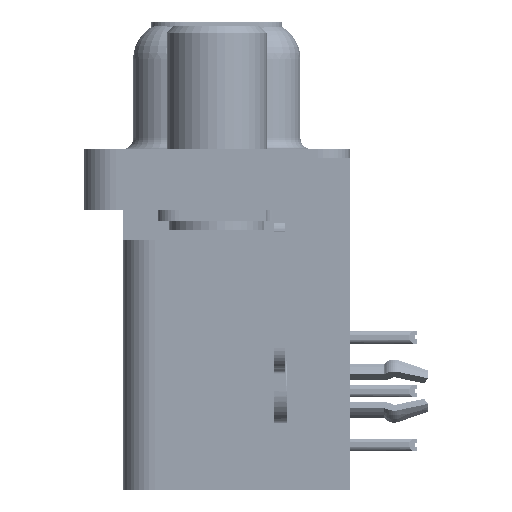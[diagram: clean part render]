
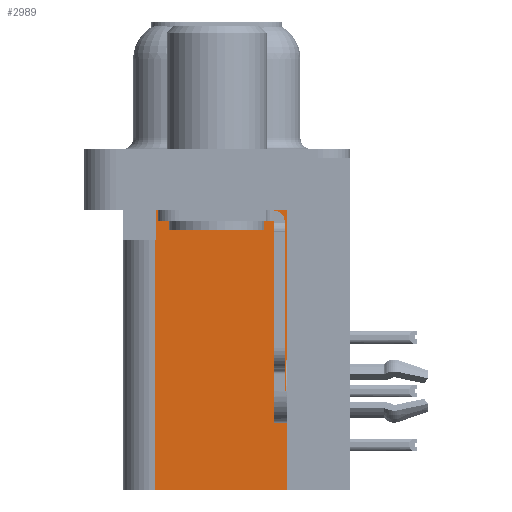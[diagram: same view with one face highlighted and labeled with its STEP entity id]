
A CAD part, left-side view. The second image highlights one B-rep face of the part: STEP entity #2989.
In plain terms, the highlighted planar face has unit normal (-1, 0, 0).
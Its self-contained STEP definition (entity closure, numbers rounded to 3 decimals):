
#494 = VECTOR ( 'NONE', #29950, 1000. ) ;
#585 = LINE ( 'NONE', #4386, #494 ) ;
#861 = CARTESIAN_POINT ( 'NONE',  ( 3.7, 2.895, -3.9 ) ) ;
#946 = CARTESIAN_POINT ( 'NONE',  ( 3.7, -3.295, -15.7 ) ) ;
#1008 = VERTEX_POINT ( 'NONE', #11969 ) ;
#2489 = ORIENTED_EDGE ( 'NONE', *, *, #38398, .F. ) ;
#2519 = ORIENTED_EDGE ( 'NONE', *, *, #19149, .T. ) ;
#2989 = ADVANCED_FACE ( 'NONE', ( #27895 ), #31195, .F. ) ;
#3293 = CARTESIAN_POINT ( 'NONE',  ( 3.7, 2.925, -15.7 ) ) ;
#4056 = DIRECTION ( 'NONE',  ( 0., 0., -1. ) ) ;
#4386 = CARTESIAN_POINT ( 'NONE',  ( 3.7, 0., -3.9 ) ) ;
#7156 = CARTESIAN_POINT ( 'NONE',  ( 3.7, -3.295, -2.5 ) ) ;
#8198 = DIRECTION ( 'NONE',  ( 1., 0., 0. ) ) ;
#8370 = VERTEX_POINT ( 'NONE', #27624 ) ;
#10410 = EDGE_LOOP ( 'NONE', ( #25423, #2519, #21178, #13948, #2489, #39483 ) ) ;
#11108 = CARTESIAN_POINT ( 'NONE',  ( 3.7, -3.295, -15.7 ) ) ;
#11461 = VERTEX_POINT ( 'NONE', #7156 ) ;
#11969 = CARTESIAN_POINT ( 'NONE',  ( 3.7, 2.925, -3.9 ) ) ;
#12311 = LINE ( 'NONE', #946, #14527 ) ;
#13385 = AXIS2_PLACEMENT_3D ( 'NONE', #24104, #8198, #4056 ) ;
#13948 = ORIENTED_EDGE ( 'NONE', *, *, #35701, .F. ) ;
#14527 = VECTOR ( 'NONE', #44379, 1000. ) ;
#15742 = DIRECTION ( 'NONE',  ( 0., 0., -1. ) ) ;
#16712 = EDGE_CURVE ( 'NONE', #11461, #39770, #20720, .T. ) ;
#17461 = VERTEX_POINT ( 'NONE', #31214 ) ;
#18276 = VECTOR ( 'NONE', #39892, 1000. ) ;
#18320 = LINE ( 'NONE', #11108, #18276 ) ;
#19149 = EDGE_CURVE ( 'NONE', #39770, #8370, #33624, .T. ) ;
#20395 = VECTOR ( 'NONE', #43331, 1000. ) ;
#20720 = LINE ( 'NONE', #25083, #20395 ) ;
#21178 = ORIENTED_EDGE ( 'NONE', *, *, #22299, .T. ) ;
#22299 = EDGE_CURVE ( 'NONE', #8370, #1008, #585, .T. ) ;
#24104 = CARTESIAN_POINT ( 'NONE',  ( 3.7, -3.295, -15.7 ) ) ;
#24733 = VERTEX_POINT ( 'NONE', #27742 ) ;
#25083 = CARTESIAN_POINT ( 'NONE',  ( 3.7, -3.295, -2.5 ) ) ;
#25423 = ORIENTED_EDGE ( 'NONE', *, *, #16712, .T. ) ;
#27624 = CARTESIAN_POINT ( 'NONE',  ( 3.7, 2.895, -3.9 ) ) ;
#27742 = CARTESIAN_POINT ( 'NONE',  ( 3.7, 2.925, -15.7 ) ) ;
#27895 = FACE_OUTER_BOUND ( 'NONE', #10410, .T. ) ;
#28932 = DIRECTION ( 'NONE',  ( 0., 0., 1. ) ) ;
#29950 = DIRECTION ( 'NONE',  ( 0., 1., 0. ) ) ;
#31195 = PLANE ( 'NONE',  #13385 ) ;
#31214 = CARTESIAN_POINT ( 'NONE',  ( 3.7, -3.295, -15.7 ) ) ;
#33624 = LINE ( 'NONE', #861, #33776 ) ;
#33776 = VECTOR ( 'NONE', #15742, 1000. ) ;
#35701 = EDGE_CURVE ( 'NONE', #24733, #1008, #41356, .T. ) ;
#38398 = EDGE_CURVE ( 'NONE', #17461, #24733, #18320, .T. ) ;
#39137 = EDGE_CURVE ( 'NONE', #17461, #11461, #12311, .T. ) ;
#39483 = ORIENTED_EDGE ( 'NONE', *, *, #39137, .T. ) ;
#39770 = VERTEX_POINT ( 'NONE', #44278 ) ;
#39892 = DIRECTION ( 'NONE',  ( 0., 1., 0. ) ) ;
#41356 = LINE ( 'NONE', #3293, #41803 ) ;
#41803 = VECTOR ( 'NONE', #28932, 1000. ) ;
#43331 = DIRECTION ( 'NONE',  ( 0., 1., 0. ) ) ;
#44278 = CARTESIAN_POINT ( 'NONE',  ( 3.7, 2.895, -2.5 ) ) ;
#44379 = DIRECTION ( 'NONE',  ( 0., 0., 1. ) ) ;
